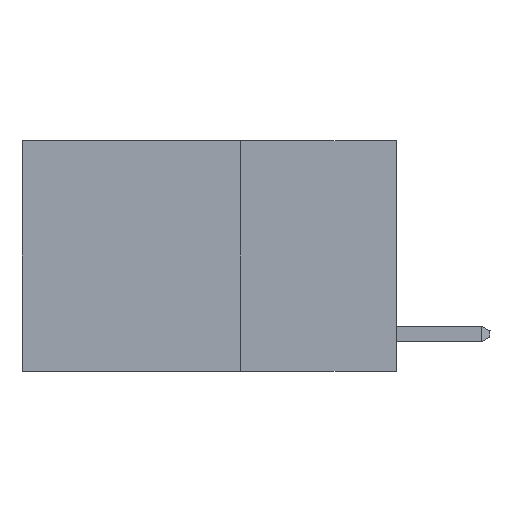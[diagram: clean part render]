
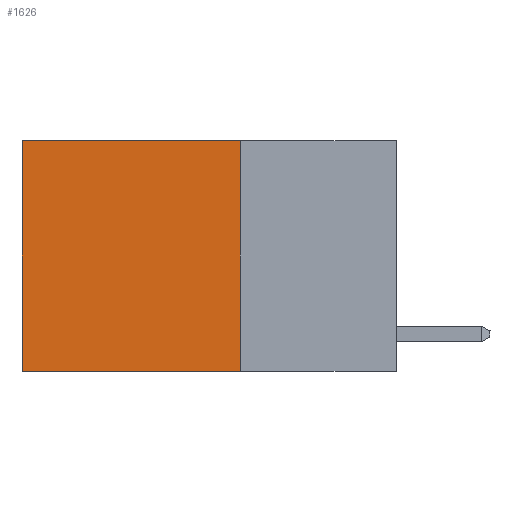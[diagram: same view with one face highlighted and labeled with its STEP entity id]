
A CAD part, left-side view. The second image highlights one B-rep face of the part: STEP entity #1626.
In plain terms, the highlighted planar face has unit normal (-1, 0, 0).
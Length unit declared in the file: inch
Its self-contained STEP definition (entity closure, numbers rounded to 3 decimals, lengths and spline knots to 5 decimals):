
#290 = VECTOR ( 'NONE', #7103, 39.37008 ) ;
#934 = DIRECTION ( 'NONE',  ( 0., 0., -1. ) ) ;
#1563 = EDGE_LOOP ( 'NONE', ( #18084, #3589, #16950, #18504 ) ) ;
#1626 = ADVANCED_FACE ( 'NONE', ( #6284 ), #12365, .F. ) ;
#1864 = EDGE_CURVE ( 'NONE', #9343, #9889, #2584, .T. ) ;
#2110 = VECTOR ( 'NONE', #8367, 39.37008 ) ;
#2422 = AXIS2_PLACEMENT_3D ( 'NONE', #18466, #13574, #18174 ) ;
#2584 = LINE ( 'NONE', #11853, #2110 ) ;
#2596 = CARTESIAN_POINT ( 'NONE',  ( 0.2625, 0.6, 0. ) ) ;
#3589 = ORIENTED_EDGE ( 'NONE', *, *, #1864, .F. ) ;
#5852 = CARTESIAN_POINT ( 'NONE',  ( 0.2625, 0.25, 0. ) ) ;
#6284 = FACE_OUTER_BOUND ( 'NONE', #1563, .T. ) ;
#6417 = VECTOR ( 'NONE', #934, 39.37008 ) ;
#7011 = LINE ( 'NONE', #13396, #290 ) ;
#7088 = CARTESIAN_POINT ( 'NONE',  ( 0.2625, 0.25, -0.37 ) ) ;
#7103 = DIRECTION ( 'NONE',  ( 0., 1., 0. ) ) ;
#7628 = EDGE_CURVE ( 'NONE', #17577, #9343, #19198, .T. ) ;
#8367 = DIRECTION ( 'NONE',  ( 0., 1., 0. ) ) ;
#8816 = CARTESIAN_POINT ( 'NONE',  ( 0.2625, 0.6, -0.37 ) ) ;
#9343 = VERTEX_POINT ( 'NONE', #7088 ) ;
#9362 = EDGE_CURVE ( 'NONE', #10268, #9889, #10159, .T. ) ;
#9889 = VERTEX_POINT ( 'NONE', #8816 ) ;
#10159 = LINE ( 'NONE', #2596, #17000 ) ;
#10268 = VERTEX_POINT ( 'NONE', #14703 ) ;
#11853 = CARTESIAN_POINT ( 'NONE',  ( 0.2625, 0.25, -0.37 ) ) ;
#12365 = PLANE ( 'NONE',  #2422 ) ;
#13396 = CARTESIAN_POINT ( 'NONE',  ( 0.2625, 0.25, 0. ) ) ;
#13574 = DIRECTION ( 'NONE',  ( 1., 0., 0. ) ) ;
#14703 = CARTESIAN_POINT ( 'NONE',  ( 0.2625, 0.6, 0. ) ) ;
#16103 = CARTESIAN_POINT ( 'NONE',  ( 0.2625, 0.25, 0. ) ) ;
#16281 = DIRECTION ( 'NONE',  ( 0., 0., -1. ) ) ;
#16489 = EDGE_CURVE ( 'NONE', #17577, #10268, #7011, .T. ) ;
#16950 = ORIENTED_EDGE ( 'NONE', *, *, #7628, .F. ) ;
#17000 = VECTOR ( 'NONE', #16281, 39.37008 ) ;
#17577 = VERTEX_POINT ( 'NONE', #5852 ) ;
#18084 = ORIENTED_EDGE ( 'NONE', *, *, #9362, .T. ) ;
#18174 = DIRECTION ( 'NONE',  ( 0., 0., -1. ) ) ;
#18466 = CARTESIAN_POINT ( 'NONE',  ( 0.2625, 0.25, 0. ) ) ;
#18504 = ORIENTED_EDGE ( 'NONE', *, *, #16489, .T. ) ;
#19198 = LINE ( 'NONE', #16103, #6417 ) ;
